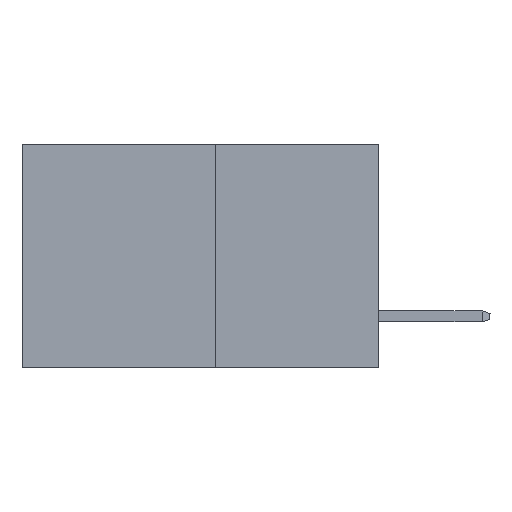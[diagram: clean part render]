
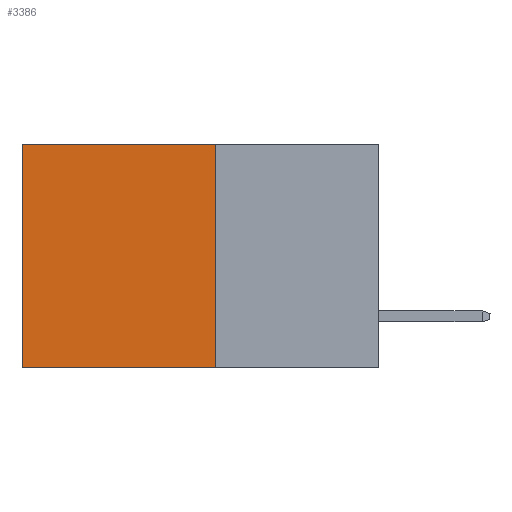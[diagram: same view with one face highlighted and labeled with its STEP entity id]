
A CAD part, left-side view. The second image highlights one B-rep face of the part: STEP entity #3386.
In plain terms, the highlighted planar face has unit normal (-1, 0, 0).
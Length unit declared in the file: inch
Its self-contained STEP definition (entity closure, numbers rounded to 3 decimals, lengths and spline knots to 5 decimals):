
#68 = CARTESIAN_POINT ( 'NONE',  ( 0.277, 0.59, -0.37 ) ) ;
#138 = VERTEX_POINT ( 'NONE', #8840 ) ;
#432 = DIRECTION ( 'NONE',  ( 0., 1., 0. ) ) ;
#544 = CARTESIAN_POINT ( 'NONE',  ( 0.277, 0.27, -0.37 ) ) ;
#1266 = CARTESIAN_POINT ( 'NONE',  ( 0.277, 0.59, -0.37 ) ) ;
#1312 = CARTESIAN_POINT ( 'NONE',  ( 0.277, 0.27, 0. ) ) ;
#2505 = ORIENTED_EDGE ( 'NONE', *, *, #8401, .F. ) ;
#3061 = AXIS2_PLACEMENT_3D ( 'NONE', #9698, #7324, #7083 ) ;
#3386 = ADVANCED_FACE ( 'NONE', ( #6712 ), #10833, .F. ) ;
#4483 = LINE ( 'NONE', #1266, #8519 ) ;
#4532 = VECTOR ( 'NONE', #9202, 39.37008 ) ;
#5123 = VERTEX_POINT ( 'NONE', #1312 ) ;
#5210 = EDGE_CURVE ( 'NONE', #138, #5247, #11028, .T. ) ;
#5247 = VERTEX_POINT ( 'NONE', #68 ) ;
#5333 = CARTESIAN_POINT ( 'NONE',  ( 0.277, 0.27, 0. ) ) ;
#5436 = ORIENTED_EDGE ( 'NONE', *, *, #5210, .F. ) ;
#6034 = LINE ( 'NONE', #7989, #9548 ) ;
#6367 = EDGE_CURVE ( 'NONE', #9193, #5247, #4483, .T. ) ;
#6712 = FACE_OUTER_BOUND ( 'NONE', #9551, .T. ) ;
#7052 = CARTESIAN_POINT ( 'NONE',  ( 0.277, 0.59, 0. ) ) ;
#7082 = ORIENTED_EDGE ( 'NONE', *, *, #7368, .T. ) ;
#7083 = DIRECTION ( 'NONE',  ( 0., 0., -1. ) ) ;
#7324 = DIRECTION ( 'NONE',  ( 1., 0., 0. ) ) ;
#7368 = EDGE_CURVE ( 'NONE', #5123, #9193, #8800, .T. ) ;
#7989 = CARTESIAN_POINT ( 'NONE',  ( 0.277, 0.27, -0.37 ) ) ;
#8401 = EDGE_CURVE ( 'NONE', #5123, #138, #6034, .T. ) ;
#8519 = VECTOR ( 'NONE', #9154, 39.37008 ) ;
#8708 = DIRECTION ( 'NONE',  ( 0., 0., -1. ) ) ;
#8800 = LINE ( 'NONE', #5333, #4532 ) ;
#8840 = CARTESIAN_POINT ( 'NONE',  ( 0.277, 0.27, -0.37 ) ) ;
#9115 = VECTOR ( 'NONE', #432, 39.37008 ) ;
#9154 = DIRECTION ( 'NONE',  ( 0., 0., -1. ) ) ;
#9193 = VERTEX_POINT ( 'NONE', #7052 ) ;
#9202 = DIRECTION ( 'NONE',  ( 0., 1., 0. ) ) ;
#9548 = VECTOR ( 'NONE', #8708, 39.37008 ) ;
#9551 = EDGE_LOOP ( 'NONE', ( #10575, #5436, #2505, #7082 ) ) ;
#9698 = CARTESIAN_POINT ( 'NONE',  ( 0.277, 0.27, -0.37 ) ) ;
#10575 = ORIENTED_EDGE ( 'NONE', *, *, #6367, .T. ) ;
#10833 = PLANE ( 'NONE',  #3061 ) ;
#11028 = LINE ( 'NONE', #544, #9115 ) ;
